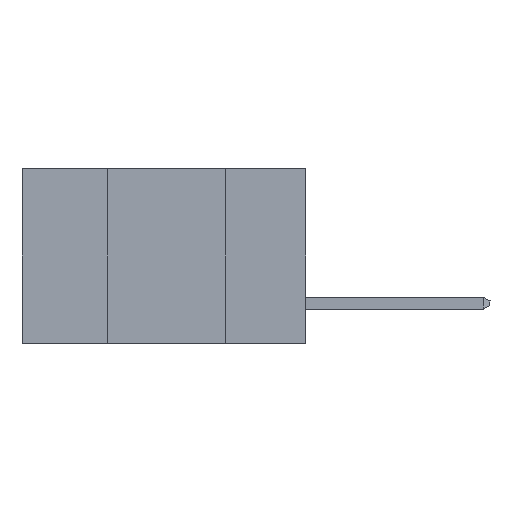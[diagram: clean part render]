
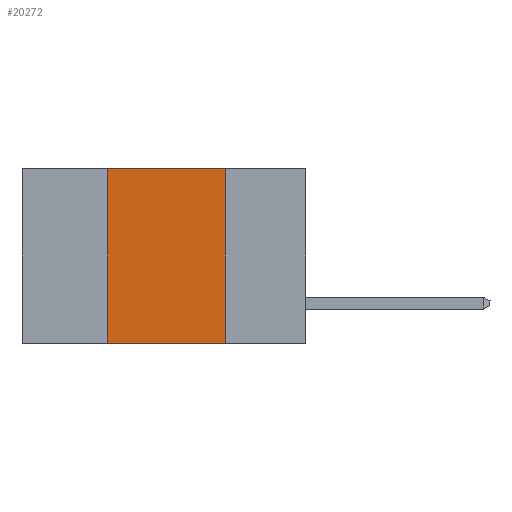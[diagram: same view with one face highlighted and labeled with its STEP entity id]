
A CAD part, left-side view. The second image highlights one B-rep face of the part: STEP entity #20272.
In plain terms, the highlighted planar face has unit normal (-1, 0, 0).
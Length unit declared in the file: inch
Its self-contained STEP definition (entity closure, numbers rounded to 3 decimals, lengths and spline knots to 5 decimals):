
#1762 = EDGE_CURVE ( 'NONE', #23261, #17282, #25358, .T. ) ;
#1785 = CARTESIAN_POINT ( 'NONE',  ( 0., 0.42, -0.37 ) ) ;
#2631 = CARTESIAN_POINT ( 'NONE',  ( 0., 0.17, 0. ) ) ;
#3391 = VECTOR ( 'NONE', #16663, 39.37008 ) ;
#3817 = DIRECTION ( 'NONE',  ( 0., 0., 1. ) ) ;
#4923 = ORIENTED_EDGE ( 'NONE', *, *, #1762, .F. ) ;
#5316 = CARTESIAN_POINT ( 'NONE',  ( 0., 0.6, 0. ) ) ;
#5372 = CARTESIAN_POINT ( 'NONE',  ( 0., 0.42, 0. ) ) ;
#5401 = FACE_OUTER_BOUND ( 'NONE', #16881, .T. ) ;
#5805 = CARTESIAN_POINT ( 'NONE',  ( 0., 0.17, 0. ) ) ;
#7423 = DIRECTION ( 'NONE',  ( 1., 0., 0. ) ) ;
#7486 = AXIS2_PLACEMENT_3D ( 'NONE', #5316, #7423, #7690 ) ;
#7690 = DIRECTION ( 'NONE',  ( 0., 0., -1. ) ) ;
#8130 = ORIENTED_EDGE ( 'NONE', *, *, #11007, .F. ) ;
#9239 = ORIENTED_EDGE ( 'NONE', *, *, #16222, .T. ) ;
#9642 = PLANE ( 'NONE',  #7486 ) ;
#11007 = EDGE_CURVE ( 'NONE', #13737, #23261, #13663, .T. ) ;
#12185 = CARTESIAN_POINT ( 'NONE',  ( 0., 0.6, 0. ) ) ;
#12451 = CARTESIAN_POINT ( 'NONE',  ( 0., 0.42, 0. ) ) ;
#12557 = VECTOR ( 'NONE', #14983, 39.37008 ) ;
#13076 = VERTEX_POINT ( 'NONE', #17118 ) ;
#13087 = ORIENTED_EDGE ( 'NONE', *, *, #17889, .F. ) ;
#13365 = VECTOR ( 'NONE', #3817, 39.37008 ) ;
#13663 = LINE ( 'NONE', #5372, #13365 ) ;
#13737 = VERTEX_POINT ( 'NONE', #1785 ) ;
#14323 = VECTOR ( 'NONE', #14739, 39.37008 ) ;
#14653 = CARTESIAN_POINT ( 'NONE',  ( 0., 0.6, -0.37 ) ) ;
#14739 = DIRECTION ( 'NONE',  ( 0., -1., 0. ) ) ;
#14983 = DIRECTION ( 'NONE',  ( 0., 0., -1. ) ) ;
#16222 = EDGE_CURVE ( 'NONE', #13737, #13076, #19204, .T. ) ;
#16663 = DIRECTION ( 'NONE',  ( 0., -1., 0. ) ) ;
#16881 = EDGE_LOOP ( 'NONE', ( #13087, #4923, #8130, #9239 ) ) ;
#17118 = CARTESIAN_POINT ( 'NONE',  ( 0., 0.17, -0.37 ) ) ;
#17282 = VERTEX_POINT ( 'NONE', #5805 ) ;
#17889 = EDGE_CURVE ( 'NONE', #17282, #13076, #25952, .T. ) ;
#19204 = LINE ( 'NONE', #14653, #14323 ) ;
#20272 = ADVANCED_FACE ( 'NONE', ( #5401 ), #9642, .F. ) ;
#23261 = VERTEX_POINT ( 'NONE', #12451 ) ;
#25358 = LINE ( 'NONE', #12185, #3391 ) ;
#25952 = LINE ( 'NONE', #2631, #12557 ) ;
